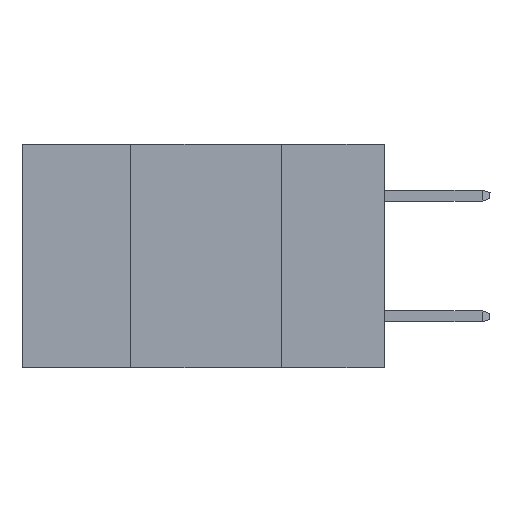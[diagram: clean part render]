
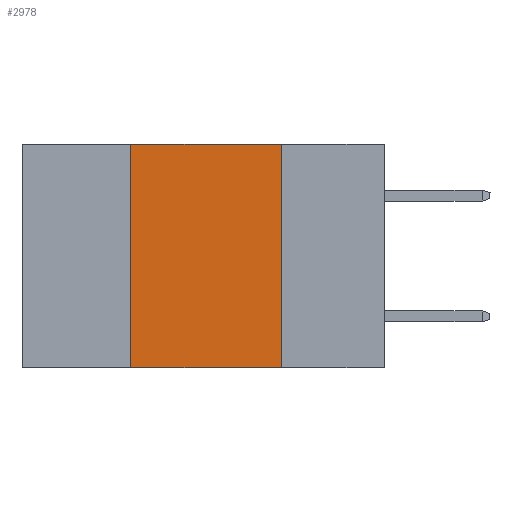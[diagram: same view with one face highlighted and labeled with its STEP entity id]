
A CAD part, left-side view. The second image highlights one B-rep face of the part: STEP entity #2978.
In plain terms, the highlighted planar face has unit normal (-1, 0, 0).
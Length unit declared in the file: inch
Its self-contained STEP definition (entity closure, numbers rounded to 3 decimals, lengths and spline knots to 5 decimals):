
#407 = DIRECTION ( 'NONE',  ( 0., -1., 0. ) ) ;
#779 = LINE ( 'NONE', #10618, #1303 ) ;
#920 = CARTESIAN_POINT ( 'NONE',  ( 0., 0.42, 0. ) ) ;
#950 = ORIENTED_EDGE ( 'NONE', *, *, #2745, .T. ) ;
#1263 = CARTESIAN_POINT ( 'NONE',  ( 0., 0.17, 0. ) ) ;
#1281 = VERTEX_POINT ( 'NONE', #5964 ) ;
#1303 = VECTOR ( 'NONE', #4114, 39.37008 ) ;
#1824 = ORIENTED_EDGE ( 'NONE', *, *, #7165, .F. ) ;
#1831 = DIRECTION ( 'NONE',  ( 0., -1., 0. ) ) ;
#2714 = VERTEX_POINT ( 'NONE', #5157 ) ;
#2734 = VERTEX_POINT ( 'NONE', #920 ) ;
#2745 = EDGE_CURVE ( 'NONE', #1281, #2714, #5321, .T. ) ;
#2978 = ADVANCED_FACE ( 'NONE', ( #10163 ), #8870, .F. ) ;
#3125 = EDGE_CURVE ( 'NONE', #3248, #2714, #5166, .T. ) ;
#3248 = VERTEX_POINT ( 'NONE', #1263 ) ;
#3488 = CARTESIAN_POINT ( 'NONE',  ( 0., 0.17, 0. ) ) ;
#4114 = DIRECTION ( 'NONE',  ( 0., 0., 1. ) ) ;
#4941 = LINE ( 'NONE', #8801, #5332 ) ;
#5027 = VECTOR ( 'NONE', #9348, 39.37008 ) ;
#5157 = CARTESIAN_POINT ( 'NONE',  ( 0., 0.17, -0.37 ) ) ;
#5166 = LINE ( 'NONE', #3488, #5027 ) ;
#5321 = LINE ( 'NONE', #6719, #7767 ) ;
#5332 = VECTOR ( 'NONE', #407, 39.37008 ) ;
#5455 = CARTESIAN_POINT ( 'NONE',  ( 0., 0.6, 0. ) ) ;
#5530 = DIRECTION ( 'NONE',  ( 1., 0., 0. ) ) ;
#5961 = EDGE_LOOP ( 'NONE', ( #9853, #8735, #1824, #950 ) ) ;
#5964 = CARTESIAN_POINT ( 'NONE',  ( 0., 0.42, -0.37 ) ) ;
#6719 = CARTESIAN_POINT ( 'NONE',  ( 0., 0.6, -0.37 ) ) ;
#7165 = EDGE_CURVE ( 'NONE', #1281, #2734, #779, .T. ) ;
#7767 = VECTOR ( 'NONE', #1831, 39.37008 ) ;
#8735 = ORIENTED_EDGE ( 'NONE', *, *, #9264, .F. ) ;
#8801 = CARTESIAN_POINT ( 'NONE',  ( 0., 0.6, 0. ) ) ;
#8870 = PLANE ( 'NONE',  #9159 ) ;
#9159 = AXIS2_PLACEMENT_3D ( 'NONE', #5455, #5530, #9681 ) ;
#9264 = EDGE_CURVE ( 'NONE', #2734, #3248, #4941, .T. ) ;
#9348 = DIRECTION ( 'NONE',  ( 0., 0., -1. ) ) ;
#9681 = DIRECTION ( 'NONE',  ( 0., 0., -1. ) ) ;
#9853 = ORIENTED_EDGE ( 'NONE', *, *, #3125, .F. ) ;
#10163 = FACE_OUTER_BOUND ( 'NONE', #5961, .T. ) ;
#10618 = CARTESIAN_POINT ( 'NONE',  ( 0., 0.42, 0. ) ) ;
